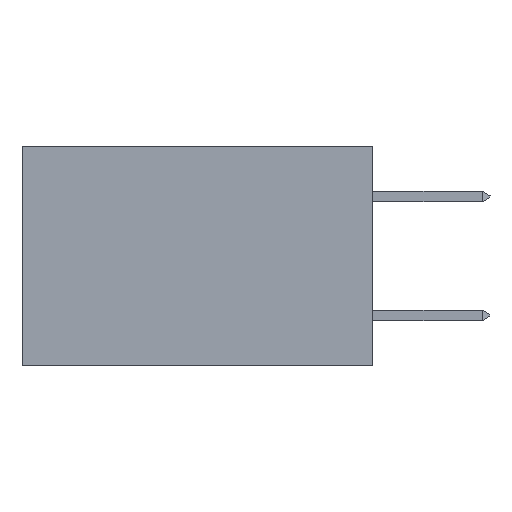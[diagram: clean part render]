
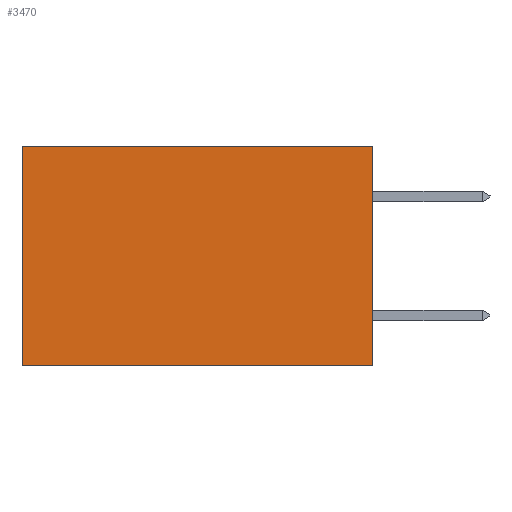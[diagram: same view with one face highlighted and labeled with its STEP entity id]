
A CAD part, left-side view. The second image highlights one B-rep face of the part: STEP entity #3470.
In plain terms, the highlighted planar face has unit normal (-1, 0, 0).
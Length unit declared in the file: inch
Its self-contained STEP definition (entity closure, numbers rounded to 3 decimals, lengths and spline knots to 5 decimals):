
#278 = CARTESIAN_POINT ( 'NONE',  ( 0.277, 0.59, -0.37 ) ) ;
#406 = CARTESIAN_POINT ( 'NONE',  ( 0.277, 0.59, 0. ) ) ;
#788 = EDGE_LOOP ( 'NONE', ( #17258, #4240, #14707, #11843 ) ) ;
#1294 = CARTESIAN_POINT ( 'NONE',  ( 0.277, 0., -0.37 ) ) ;
#1330 = AXIS2_PLACEMENT_3D ( 'NONE', #9206, #8965, #7957 ) ;
#1485 = DIRECTION ( 'NONE',  ( 0., 0., -1. ) ) ;
#1886 = CARTESIAN_POINT ( 'NONE',  ( 0.277, 0., -0.37 ) ) ;
#2592 = CARTESIAN_POINT ( 'NONE',  ( 0.277, 0.59, -0.37 ) ) ;
#3016 = VERTEX_POINT ( 'NONE', #2592 ) ;
#3470 = ADVANCED_FACE ( 'NONE', ( #13330 ), #9194, .F. ) ;
#3643 = EDGE_CURVE ( 'NONE', #10406, #15612, #7410, .T. ) ;
#3716 = VECTOR ( 'NONE', #1485, 39.37008 ) ;
#3872 = EDGE_CURVE ( 'NONE', #10406, #17628, #11306, .T. ) ;
#4240 = ORIENTED_EDGE ( 'NONE', *, *, #12284, .F. ) ;
#4658 = VECTOR ( 'NONE', #14218, 39.37008 ) ;
#7410 = LINE ( 'NONE', #1294, #3716 ) ;
#7621 = VECTOR ( 'NONE', #13702, 39.37008 ) ;
#7957 = DIRECTION ( 'NONE',  ( 0., 0., -1. ) ) ;
#8965 = DIRECTION ( 'NONE',  ( 1., 0., 0. ) ) ;
#9194 = PLANE ( 'NONE',  #1330 ) ;
#9206 = CARTESIAN_POINT ( 'NONE',  ( 0.277, 0., -0.37 ) ) ;
#9366 = VECTOR ( 'NONE', #15352, 39.37008 ) ;
#10406 = VERTEX_POINT ( 'NONE', #11709 ) ;
#11060 = CARTESIAN_POINT ( 'NONE',  ( 0.277, 0., -0.37 ) ) ;
#11306 = LINE ( 'NONE', #13365, #7621 ) ;
#11709 = CARTESIAN_POINT ( 'NONE',  ( 0.277, 0., 0. ) ) ;
#11843 = ORIENTED_EDGE ( 'NONE', *, *, #3872, .T. ) ;
#12033 = LINE ( 'NONE', #278, #4658 ) ;
#12284 = EDGE_CURVE ( 'NONE', #15612, #3016, #16358, .T. ) ;
#13330 = FACE_OUTER_BOUND ( 'NONE', #788, .T. ) ;
#13365 = CARTESIAN_POINT ( 'NONE',  ( 0.277, 0., 0. ) ) ;
#13702 = DIRECTION ( 'NONE',  ( 0., 1., 0. ) ) ;
#14218 = DIRECTION ( 'NONE',  ( 0., 0., -1. ) ) ;
#14707 = ORIENTED_EDGE ( 'NONE', *, *, #3643, .F. ) ;
#15352 = DIRECTION ( 'NONE',  ( 0., 1., 0. ) ) ;
#15612 = VERTEX_POINT ( 'NONE', #1886 ) ;
#16358 = LINE ( 'NONE', #11060, #9366 ) ;
#17258 = ORIENTED_EDGE ( 'NONE', *, *, #17549, .T. ) ;
#17549 = EDGE_CURVE ( 'NONE', #17628, #3016, #12033, .T. ) ;
#17628 = VERTEX_POINT ( 'NONE', #406 ) ;
